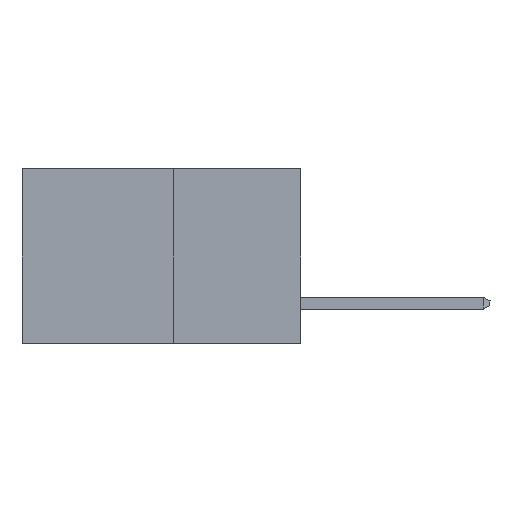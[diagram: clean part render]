
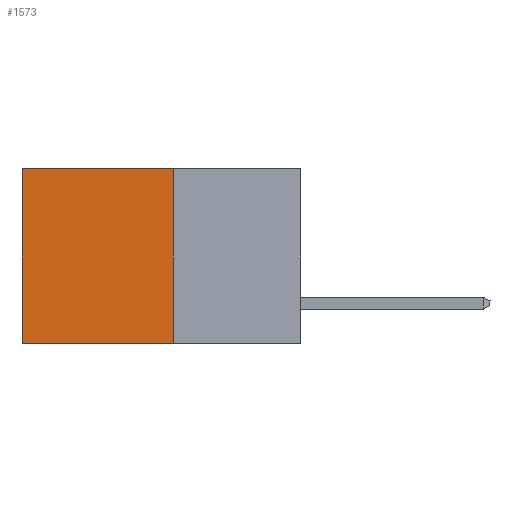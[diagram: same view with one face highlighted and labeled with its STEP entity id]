
A CAD part, left-side view. The second image highlights one B-rep face of the part: STEP entity #1573.
In plain terms, the highlighted planar face has unit normal (-1, 0, 0).
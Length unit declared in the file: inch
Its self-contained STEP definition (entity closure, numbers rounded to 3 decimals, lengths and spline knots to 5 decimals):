
#70 = VERTEX_POINT ( 'NONE', #1363 ) ;
#882 = EDGE_CURVE ( 'NONE', #10489, #70, #5474, .T. ) ;
#1046 = VERTEX_POINT ( 'NONE', #5407 ) ;
#1112 = CARTESIAN_POINT ( 'NONE',  ( 0.277, 0.27, -0.37 ) ) ;
#1234 = LINE ( 'NONE', #5889, #9566 ) ;
#1330 = CARTESIAN_POINT ( 'NONE',  ( 0.277, 0.27, 0. ) ) ;
#1363 = CARTESIAN_POINT ( 'NONE',  ( 0.277, 0.59, -0.37 ) ) ;
#1422 = PLANE ( 'NONE',  #10067 ) ;
#1546 = EDGE_CURVE ( 'NONE', #1046, #70, #1234, .T. ) ;
#1573 = ADVANCED_FACE ( 'NONE', ( #3905 ), #1422, .F. ) ;
#2100 = DIRECTION ( 'NONE',  ( 0., 0., -1. ) ) ;
#2627 = CARTESIAN_POINT ( 'NONE',  ( 0.277, 0.27, -0.37 ) ) ;
#3051 = CARTESIAN_POINT ( 'NONE',  ( 0.277, 0.27, -0.37 ) ) ;
#3472 = EDGE_CURVE ( 'NONE', #8470, #10489, #4721, .T. ) ;
#3905 = FACE_OUTER_BOUND ( 'NONE', #10011, .T. ) ;
#4529 = DIRECTION ( 'NONE',  ( 0., 1., 0. ) ) ;
#4721 = LINE ( 'NONE', #2627, #9648 ) ;
#5407 = CARTESIAN_POINT ( 'NONE',  ( 0.277, 0.59, 0. ) ) ;
#5474 = LINE ( 'NONE', #3051, #12725 ) ;
#5684 = ORIENTED_EDGE ( 'NONE', *, *, #3472, .F. ) ;
#5889 = CARTESIAN_POINT ( 'NONE',  ( 0.277, 0.59, -0.37 ) ) ;
#6529 = DIRECTION ( 'NONE',  ( 1., 0., 0. ) ) ;
#8371 = DIRECTION ( 'NONE',  ( 0., 0., -1. ) ) ;
#8470 = VERTEX_POINT ( 'NONE', #1330 ) ;
#9566 = VECTOR ( 'NONE', #12361, 39.37008 ) ;
#9648 = VECTOR ( 'NONE', #2100, 39.37008 ) ;
#9808 = VECTOR ( 'NONE', #11964, 39.37008 ) ;
#9828 = CARTESIAN_POINT ( 'NONE',  ( 0.277, 0.27, -0.37 ) ) ;
#10011 = EDGE_LOOP ( 'NONE', ( #12926, #13215, #5684, #13541 ) ) ;
#10067 = AXIS2_PLACEMENT_3D ( 'NONE', #1112, #6529, #8371 ) ;
#10334 = EDGE_CURVE ( 'NONE', #8470, #1046, #12466, .T. ) ;
#10489 = VERTEX_POINT ( 'NONE', #9828 ) ;
#10949 = CARTESIAN_POINT ( 'NONE',  ( 0.277, 0.27, 0. ) ) ;
#11964 = DIRECTION ( 'NONE',  ( 0., 1., 0. ) ) ;
#12361 = DIRECTION ( 'NONE',  ( 0., 0., -1. ) ) ;
#12466 = LINE ( 'NONE', #10949, #9808 ) ;
#12725 = VECTOR ( 'NONE', #4529, 39.37008 ) ;
#12926 = ORIENTED_EDGE ( 'NONE', *, *, #1546, .T. ) ;
#13215 = ORIENTED_EDGE ( 'NONE', *, *, #882, .F. ) ;
#13541 = ORIENTED_EDGE ( 'NONE', *, *, #10334, .T. ) ;
